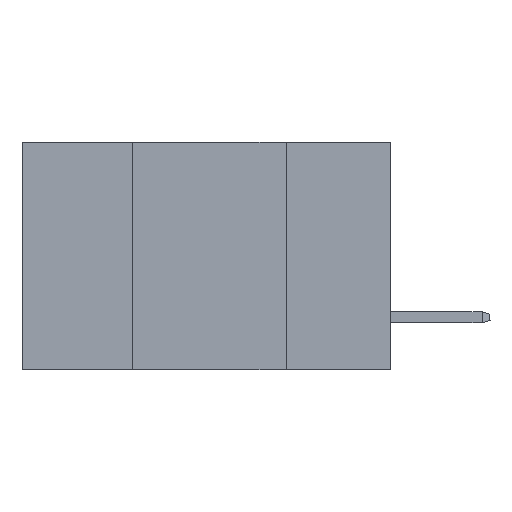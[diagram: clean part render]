
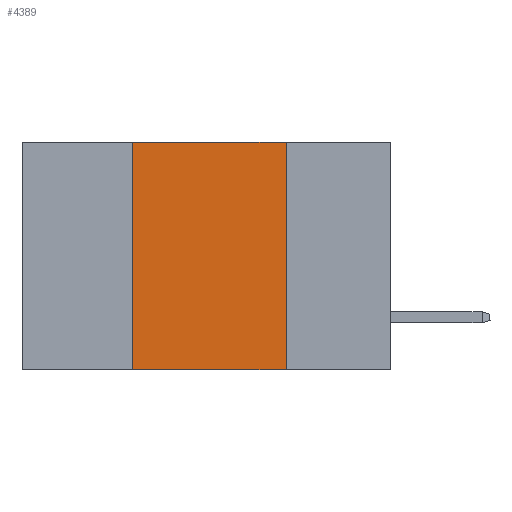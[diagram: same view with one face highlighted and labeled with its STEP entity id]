
A CAD part, left-side view. The second image highlights one B-rep face of the part: STEP entity #4389.
In plain terms, the highlighted planar face has unit normal (-1, 0, 0).
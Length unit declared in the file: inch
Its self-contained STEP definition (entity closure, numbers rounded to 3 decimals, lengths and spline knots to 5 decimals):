
#340 = CARTESIAN_POINT ( 'NONE',  ( 0., 0.42, 0. ) ) ;
#361 = DIRECTION ( 'NONE',  ( 0., 0., -1. ) ) ;
#514 = EDGE_CURVE ( 'NONE', #19168, #4666, #5825, .T. ) ;
#923 = EDGE_LOOP ( 'NONE', ( #13296, #10527, #15256, #15753 ) ) ;
#1176 = CARTESIAN_POINT ( 'NONE',  ( 0., 0.6, 0. ) ) ;
#2785 = DIRECTION ( 'NONE',  ( 1., 0., 0. ) ) ;
#4389 = ADVANCED_FACE ( 'NONE', ( #14346 ), #10769, .F. ) ;
#4666 = VERTEX_POINT ( 'NONE', #17770 ) ;
#5323 = VECTOR ( 'NONE', #13015, 39.37008 ) ;
#5407 = EDGE_CURVE ( 'NONE', #5762, #19168, #18245, .T. ) ;
#5762 = VERTEX_POINT ( 'NONE', #10854 ) ;
#5825 = LINE ( 'NONE', #13272, #5323 ) ;
#6708 = CARTESIAN_POINT ( 'NONE',  ( 0., 0.17, -0.37 ) ) ;
#6713 = CARTESIAN_POINT ( 'NONE',  ( 0., 0.17, 0. ) ) ;
#7351 = VECTOR ( 'NONE', #10270, 39.37008 ) ;
#7872 = LINE ( 'NONE', #8658, #7351 ) ;
#8391 = DIRECTION ( 'NONE',  ( 0., 0., 1. ) ) ;
#8658 = CARTESIAN_POINT ( 'NONE',  ( 0., 0.6, -0.37 ) ) ;
#10270 = DIRECTION ( 'NONE',  ( 0., -1., 0. ) ) ;
#10527 = ORIENTED_EDGE ( 'NONE', *, *, #514, .F. ) ;
#10769 = PLANE ( 'NONE',  #16042 ) ;
#10854 = CARTESIAN_POINT ( 'NONE',  ( 0., 0.42, -0.37 ) ) ;
#12836 = EDGE_CURVE ( 'NONE', #5762, #15879, #7872, .T. ) ;
#13015 = DIRECTION ( 'NONE',  ( 0., -1., 0. ) ) ;
#13272 = CARTESIAN_POINT ( 'NONE',  ( 0., 0.6, 0. ) ) ;
#13296 = ORIENTED_EDGE ( 'NONE', *, *, #18808, .F. ) ;
#13981 = DIRECTION ( 'NONE',  ( 0., 0., -1. ) ) ;
#14016 = CARTESIAN_POINT ( 'NONE',  ( 0., 0.42, 0. ) ) ;
#14045 = VECTOR ( 'NONE', #8391, 39.37008 ) ;
#14346 = FACE_OUTER_BOUND ( 'NONE', #923, .T. ) ;
#15256 = ORIENTED_EDGE ( 'NONE', *, *, #5407, .F. ) ;
#15753 = ORIENTED_EDGE ( 'NONE', *, *, #12836, .T. ) ;
#15879 = VERTEX_POINT ( 'NONE', #6708 ) ;
#16042 = AXIS2_PLACEMENT_3D ( 'NONE', #1176, #2785, #13981 ) ;
#17770 = CARTESIAN_POINT ( 'NONE',  ( 0., 0.17, 0. ) ) ;
#18245 = LINE ( 'NONE', #340, #14045 ) ;
#18808 = EDGE_CURVE ( 'NONE', #4666, #15879, #19566, .T. ) ;
#19095 = VECTOR ( 'NONE', #361, 39.37008 ) ;
#19168 = VERTEX_POINT ( 'NONE', #14016 ) ;
#19566 = LINE ( 'NONE', #6713, #19095 ) ;
